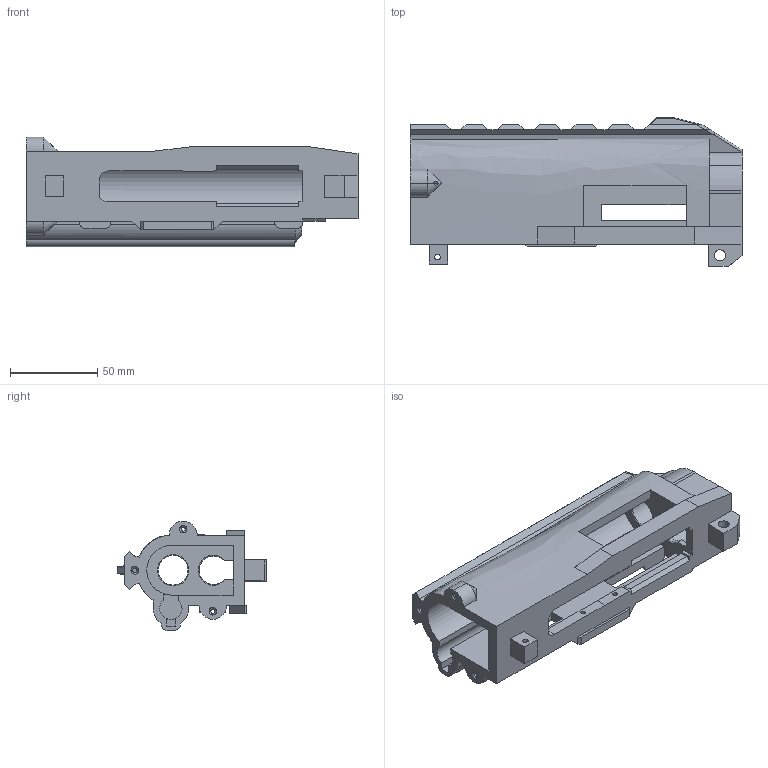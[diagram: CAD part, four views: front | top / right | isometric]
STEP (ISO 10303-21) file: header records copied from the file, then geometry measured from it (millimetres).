
FILE_DESCRIPTION(('STEP AP214'),'1');
FILE_NAME('WTF9HE Upper Receiver.stl.stp','2020-09-01T22:14:06',(' '),(' '),'Spatial InterOp 3D',' ',' ');
FILE_SCHEMA(('AUTOMOTIVE_DESIGN { 1 0 10303 214 1 1 1 1 }'));
Length unit declared in the file: metre
Products named in the file (1): Solid1
Bounding box: 190.38 x 85.37 x 62.82 mm (x, y, z)
Volume: 207973.2 mm3; surface area: 80199.8 mm2
Topology: 1 solids, 1 shells, 265 faces, 726 edges, 463 vertices
Faces by surface type: plane 157, cylinder 79, cone 21, torus 5, sphere 2, bspline 1
Entity records: 9492 total; most frequent: CARTESIAN_POINT 2629, ORIENTED_EDGE 1446, DIRECTION 1408, EDGE_CURVE 723, LINE 506, VECTOR 506, VERTEX_POINT 463, AXIS2_PLACEMENT_3D 451
